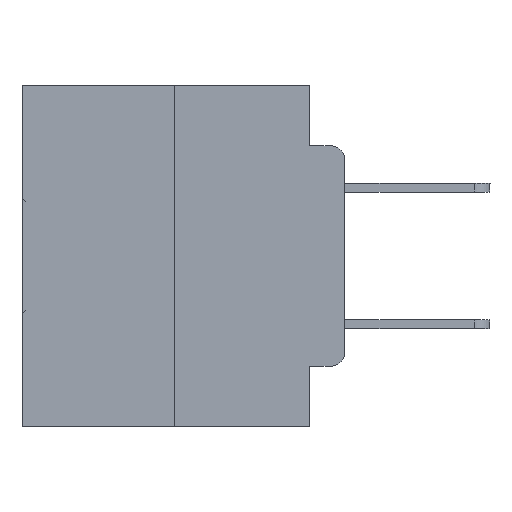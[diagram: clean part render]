
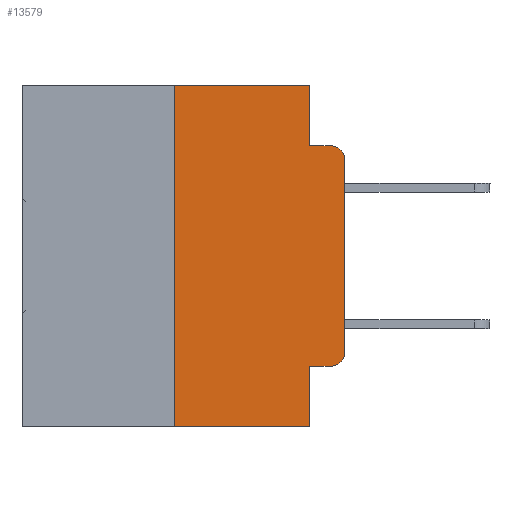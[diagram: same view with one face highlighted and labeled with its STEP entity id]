
A CAD part, left-side view. The second image highlights one B-rep face of the part: STEP entity #13579.
In plain terms, the highlighted planar face has unit normal (-1, 0, 0).
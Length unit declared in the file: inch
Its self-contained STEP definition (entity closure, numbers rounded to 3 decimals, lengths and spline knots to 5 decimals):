
#264 = EDGE_CURVE ( 'NONE', #1250, #22777, #2554, .T. ) ;
#294 = EDGE_LOOP ( 'NONE', ( #2875, #3983, #1111, #6086, #1245, #18963, #23166, #15846, #24194, #23958 ) ) ;
#297 = DIRECTION ( 'NONE',  ( 0., -1., 0. ) ) ;
#661 = CARTESIAN_POINT ( 'NONE',  ( 0., 0., -0.3915 ) ) ;
#1111 = ORIENTED_EDGE ( 'NONE', *, *, #13588, .F. ) ;
#1245 = ORIENTED_EDGE ( 'NONE', *, *, #6435, .F. ) ;
#1250 = VERTEX_POINT ( 'NONE', #23183 ) ;
#1668 = VERTEX_POINT ( 'NONE', #23662 ) ;
#2325 = CARTESIAN_POINT ( 'NONE',  ( 0., 0.051, -0.4115 ) ) ;
#2526 = CARTESIAN_POINT ( 'NONE',  ( 0., 0.051, -0.4115 ) ) ;
#2554 = CIRCLE ( 'NONE', #14898, 0.02 ) ;
#2875 = ORIENTED_EDGE ( 'NONE', *, *, #18440, .T. ) ;
#3428 = CARTESIAN_POINT ( 'NONE',  ( 0., 0.051, 0. ) ) ;
#3453 = LINE ( 'NONE', #15461, #28574 ) ;
#3636 = VECTOR ( 'NONE', #297, 39.37008 ) ;
#3983 = ORIENTED_EDGE ( 'NONE', *, *, #15215, .T. ) ;
#4371 = CARTESIAN_POINT ( 'NONE',  ( 0., 0.02, -0.1085 ) ) ;
#5322 = EDGE_CURVE ( 'NONE', #11003, #1250, #28151, .T. ) ;
#5655 = VERTEX_POINT ( 'NONE', #15907 ) ;
#5660 = CARTESIAN_POINT ( 'NONE',  ( 0., 0.02, -0.3915 ) ) ;
#5974 = DIRECTION ( 'NONE',  ( 0., 0., -1. ) ) ;
#6086 = ORIENTED_EDGE ( 'NONE', *, *, #11965, .F. ) ;
#6435 = EDGE_CURVE ( 'NONE', #14693, #12115, #13791, .T. ) ;
#6871 = LINE ( 'NONE', #27210, #31045 ) ;
#6886 = DIRECTION ( 'NONE',  ( 0., 0., -1. ) ) ;
#6977 = EDGE_CURVE ( 'NONE', #11003, #14154, #17910, .T. ) ;
#7088 = AXIS2_PLACEMENT_3D ( 'NONE', #27099, #29498, #15131 ) ;
#7719 = VECTOR ( 'NONE', #30294, 39.37008 ) ;
#7890 = EDGE_CURVE ( 'NONE', #28973, #14154, #17123, .T. ) ;
#7976 = DIRECTION ( 'NONE',  ( 0., 0., 1. ) ) ;
#8454 = CARTESIAN_POINT ( 'NONE',  ( 0., 0.473, -0.5 ) ) ;
#8513 = LINE ( 'NONE', #27940, #7719 ) ;
#8729 = CARTESIAN_POINT ( 'NONE',  ( 0., 0.02, -0.0885 ) ) ;
#9268 = CARTESIAN_POINT ( 'NONE',  ( 0., 0.051, 0. ) ) ;
#10356 = EDGE_CURVE ( 'NONE', #28973, #14693, #3453, .T. ) ;
#10523 = AXIS2_PLACEMENT_3D ( 'NONE', #4371, #21482, #6886 ) ;
#11003 = VERTEX_POINT ( 'NONE', #2526 ) ;
#11965 = EDGE_CURVE ( 'NONE', #12115, #5655, #8513, .T. ) ;
#12115 = VERTEX_POINT ( 'NONE', #9268 ) ;
#12333 = DIRECTION ( 'NONE',  ( 0., -1., 0. ) ) ;
#12694 = PLANE ( 'NONE',  #7088 ) ;
#13579 = ADVANCED_FACE ( 'NONE', ( #24624 ), #12694, .F. ) ;
#13588 = EDGE_CURVE ( 'NONE', #5655, #29939, #23123, .T. ) ;
#13791 = LINE ( 'NONE', #21027, #26584 ) ;
#14154 = VERTEX_POINT ( 'NONE', #24584 ) ;
#14693 = VERTEX_POINT ( 'NONE', #29046 ) ;
#14898 = AXIS2_PLACEMENT_3D ( 'NONE', #5660, #19776, #19872 ) ;
#15131 = DIRECTION ( 'NONE',  ( 0., 0., -1. ) ) ;
#15215 = EDGE_CURVE ( 'NONE', #1668, #29939, #21897, .T. ) ;
#15461 = CARTESIAN_POINT ( 'NONE',  ( 0., 0.25, 0. ) ) ;
#15846 = ORIENTED_EDGE ( 'NONE', *, *, #6977, .F. ) ;
#15907 = CARTESIAN_POINT ( 'NONE',  ( 0., 0.051, -0.0885 ) ) ;
#17123 = LINE ( 'NONE', #8454, #29114 ) ;
#17575 = CARTESIAN_POINT ( 'NONE',  ( 0., 0.051, -0.0885 ) ) ;
#17910 = LINE ( 'NONE', #3428, #29901 ) ;
#17970 = DIRECTION ( 'NONE',  ( 0., 0., 1. ) ) ;
#18440 = EDGE_CURVE ( 'NONE', #22777, #1668, #6871, .T. ) ;
#18963 = ORIENTED_EDGE ( 'NONE', *, *, #10356, .F. ) ;
#19710 = CARTESIAN_POINT ( 'NONE',  ( 0., 0.25, -0.5 ) ) ;
#19776 = DIRECTION ( 'NONE',  ( -1., 0., 0. ) ) ;
#19872 = DIRECTION ( 'NONE',  ( 0., 0., -1. ) ) ;
#20642 = DIRECTION ( 'NONE',  ( 0., -1., 0. ) ) ;
#21027 = CARTESIAN_POINT ( 'NONE',  ( 0., 0.473, 0. ) ) ;
#21482 = DIRECTION ( 'NONE',  ( -1., 0., 0. ) ) ;
#21775 = VECTOR ( 'NONE', #12333, 39.37008 ) ;
#21897 = CIRCLE ( 'NONE', #10523, 0.02 ) ;
#22777 = VERTEX_POINT ( 'NONE', #661 ) ;
#23123 = LINE ( 'NONE', #17575, #3636 ) ;
#23166 = ORIENTED_EDGE ( 'NONE', *, *, #7890, .T. ) ;
#23183 = CARTESIAN_POINT ( 'NONE',  ( 0., 0.02, -0.4115 ) ) ;
#23437 = DIRECTION ( 'NONE',  ( 0., -1., 0. ) ) ;
#23662 = CARTESIAN_POINT ( 'NONE',  ( 0., 0., -0.1085 ) ) ;
#23958 = ORIENTED_EDGE ( 'NONE', *, *, #264, .T. ) ;
#24194 = ORIENTED_EDGE ( 'NONE', *, *, #5322, .T. ) ;
#24584 = CARTESIAN_POINT ( 'NONE',  ( 0., 0.051, -0.5 ) ) ;
#24624 = FACE_OUTER_BOUND ( 'NONE', #294, .T. ) ;
#26584 = VECTOR ( 'NONE', #23437, 39.37008 ) ;
#27099 = CARTESIAN_POINT ( 'NONE',  ( 0., 0.473, 0. ) ) ;
#27210 = CARTESIAN_POINT ( 'NONE',  ( 0., 0., 0. ) ) ;
#27940 = CARTESIAN_POINT ( 'NONE',  ( 0., 0.051, 0. ) ) ;
#28151 = LINE ( 'NONE', #2325, #21775 ) ;
#28574 = VECTOR ( 'NONE', #17970, 39.37008 ) ;
#28973 = VERTEX_POINT ( 'NONE', #19710 ) ;
#29046 = CARTESIAN_POINT ( 'NONE',  ( 0., 0.25, 0. ) ) ;
#29114 = VECTOR ( 'NONE', #20642, 39.37008 ) ;
#29498 = DIRECTION ( 'NONE',  ( 1., 0., 0. ) ) ;
#29901 = VECTOR ( 'NONE', #5974, 39.37008 ) ;
#29939 = VERTEX_POINT ( 'NONE', #8729 ) ;
#30294 = DIRECTION ( 'NONE',  ( 0., 0., -1. ) ) ;
#31045 = VECTOR ( 'NONE', #7976, 39.37008 ) ;
